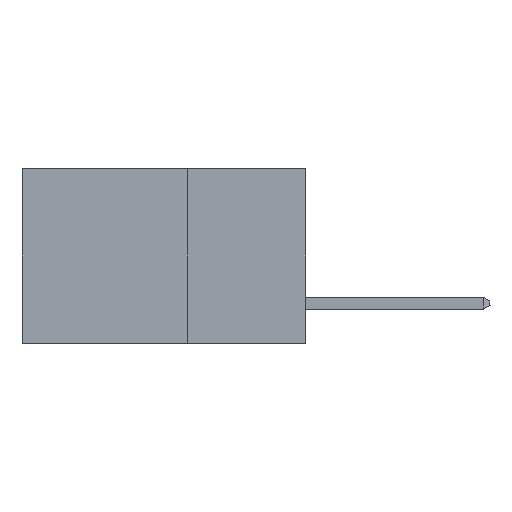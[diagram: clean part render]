
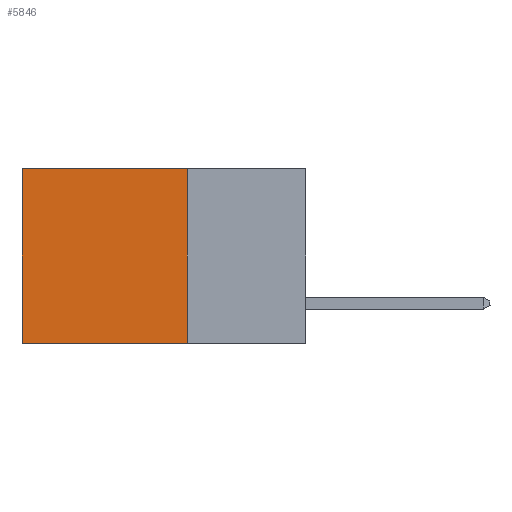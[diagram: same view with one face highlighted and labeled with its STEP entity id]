
A CAD part, left-side view. The second image highlights one B-rep face of the part: STEP entity #5846.
In plain terms, the highlighted planar face has unit normal (-1, 0, 0).
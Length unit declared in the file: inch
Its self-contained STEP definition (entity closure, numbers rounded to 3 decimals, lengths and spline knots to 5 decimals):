
#365 = CARTESIAN_POINT ( 'NONE',  ( 0.298, 0.6, -0.37 ) ) ;
#386 = EDGE_CURVE ( 'NONE', #3960, #8230, #3870, .T. ) ;
#561 = VECTOR ( 'NONE', #2579, 39.37008 ) ;
#827 = EDGE_CURVE ( 'NONE', #8230, #1536, #1098, .T. ) ;
#1098 = LINE ( 'NONE', #1239, #561 ) ;
#1239 = CARTESIAN_POINT ( 'NONE',  ( 0.298, 0.6, 0. ) ) ;
#1536 = VERTEX_POINT ( 'NONE', #365 ) ;
#1661 = VECTOR ( 'NONE', #4260, 39.37008 ) ;
#2039 = EDGE_CURVE ( 'NONE', #8492, #1536, #6388, .T. ) ;
#2053 = ORIENTED_EDGE ( 'NONE', *, *, #827, .T. ) ;
#2294 = EDGE_LOOP ( 'NONE', ( #2053, #4413, #6436, #8188 ) ) ;
#2344 = DIRECTION ( 'NONE',  ( 1., 0., 0. ) ) ;
#2579 = DIRECTION ( 'NONE',  ( 0., 0., -1. ) ) ;
#2809 = CARTESIAN_POINT ( 'NONE',  ( 0.298, 0.6, 0. ) ) ;
#3074 = DIRECTION ( 'NONE',  ( 0., 1., 0. ) ) ;
#3235 = EDGE_CURVE ( 'NONE', #3960, #8492, #7897, .T. ) ;
#3688 = CARTESIAN_POINT ( 'NONE',  ( 0.298, 0.25, 0. ) ) ;
#3870 = LINE ( 'NONE', #3688, #7804 ) ;
#3960 = VERTEX_POINT ( 'NONE', #9068 ) ;
#4260 = DIRECTION ( 'NONE',  ( 0., 0., -1. ) ) ;
#4413 = ORIENTED_EDGE ( 'NONE', *, *, #2039, .F. ) ;
#5578 = AXIS2_PLACEMENT_3D ( 'NONE', #9582, #2344, #7776 ) ;
#5846 = ADVANCED_FACE ( 'NONE', ( #8890 ), #7145, .F. ) ;
#6332 = CARTESIAN_POINT ( 'NONE',  ( 0.298, 0.25, -0.37 ) ) ;
#6388 = LINE ( 'NONE', #6332, #7936 ) ;
#6436 = ORIENTED_EDGE ( 'NONE', *, *, #3235, .F. ) ;
#7145 = PLANE ( 'NONE',  #5578 ) ;
#7765 = CARTESIAN_POINT ( 'NONE',  ( 0.298, 0.25, 0. ) ) ;
#7776 = DIRECTION ( 'NONE',  ( 0., 0., -1. ) ) ;
#7804 = VECTOR ( 'NONE', #3074, 39.37008 ) ;
#7897 = LINE ( 'NONE', #7765, #1661 ) ;
#7936 = VECTOR ( 'NONE', #8549, 39.37008 ) ;
#8188 = ORIENTED_EDGE ( 'NONE', *, *, #386, .T. ) ;
#8230 = VERTEX_POINT ( 'NONE', #2809 ) ;
#8492 = VERTEX_POINT ( 'NONE', #8752 ) ;
#8549 = DIRECTION ( 'NONE',  ( 0., 1., 0. ) ) ;
#8752 = CARTESIAN_POINT ( 'NONE',  ( 0.298, 0.25, -0.37 ) ) ;
#8890 = FACE_OUTER_BOUND ( 'NONE', #2294, .T. ) ;
#9068 = CARTESIAN_POINT ( 'NONE',  ( 0.298, 0.25, 0. ) ) ;
#9582 = CARTESIAN_POINT ( 'NONE',  ( 0.298, 0.25, 0. ) ) ;
